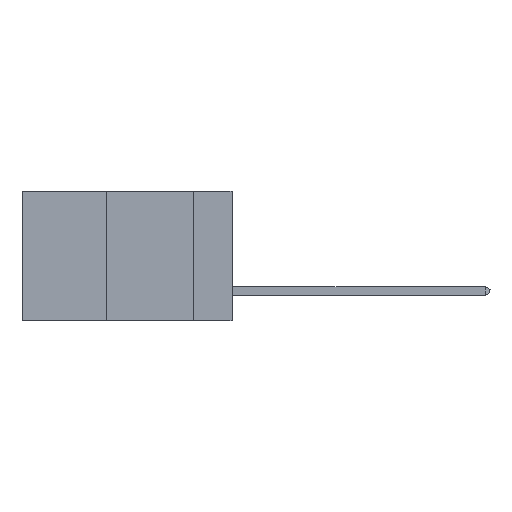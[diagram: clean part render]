
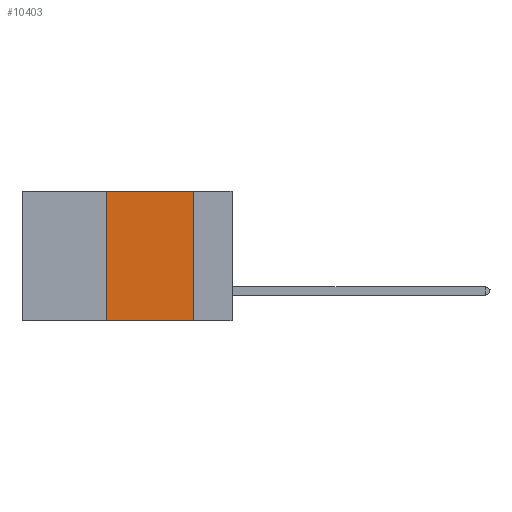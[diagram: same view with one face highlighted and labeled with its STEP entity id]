
A CAD part, left-side view. The second image highlights one B-rep face of the part: STEP entity #10403.
In plain terms, the highlighted planar face has unit normal (-1, 0, 0).
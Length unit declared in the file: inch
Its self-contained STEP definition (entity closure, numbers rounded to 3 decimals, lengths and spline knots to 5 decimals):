
#1484 = AXIS2_PLACEMENT_3D ( 'NONE', #18218, #8690, #34012 ) ;
#2479 = CARTESIAN_POINT ( 'NONE',  ( 0., 0.36, 0. ) ) ;
#2724 = CARTESIAN_POINT ( 'NONE',  ( 0., 0.6, -0.37 ) ) ;
#3680 = VERTEX_POINT ( 'NONE', #38893 ) ;
#3938 = DIRECTION ( 'NONE',  ( 0., -1., 0. ) ) ;
#5414 = VECTOR ( 'NONE', #3938, 39.37008 ) ;
#7353 = VECTOR ( 'NONE', #27477, 39.37008 ) ;
#7831 = LINE ( 'NONE', #2724, #7353 ) ;
#8361 = CARTESIAN_POINT ( 'NONE',  ( 0., 0.11, 0. ) ) ;
#8690 = DIRECTION ( 'NONE',  ( 1., 0., 0. ) ) ;
#10403 = ADVANCED_FACE ( 'NONE', ( #14463 ), #27562, .F. ) ;
#11799 = CARTESIAN_POINT ( 'NONE',  ( 0., 0.36, 0. ) ) ;
#12675 = VERTEX_POINT ( 'NONE', #37074 ) ;
#13739 = EDGE_LOOP ( 'NONE', ( #32101, #27097, #37524, #17548 ) ) ;
#14463 = FACE_OUTER_BOUND ( 'NONE', #13739, .T. ) ;
#17548 = ORIENTED_EDGE ( 'NONE', *, *, #30028, .T. ) ;
#18218 = CARTESIAN_POINT ( 'NONE',  ( 0., 0.6, 0. ) ) ;
#19046 = CARTESIAN_POINT ( 'NONE',  ( 0., 0.6, 0. ) ) ;
#19556 = EDGE_CURVE ( 'NONE', #34437, #36605, #22151, .T. ) ;
#19991 = CARTESIAN_POINT ( 'NONE',  ( 0., 0.11, 0. ) ) ;
#20805 = DIRECTION ( 'NONE',  ( 0., 0., -1. ) ) ;
#22151 = LINE ( 'NONE', #19046, #5414 ) ;
#25077 = EDGE_CURVE ( 'NONE', #12675, #34437, #33103, .T. ) ;
#27097 = ORIENTED_EDGE ( 'NONE', *, *, #19556, .F. ) ;
#27212 = VECTOR ( 'NONE', #27654, 39.37008 ) ;
#27477 = DIRECTION ( 'NONE',  ( 0., -1., 0. ) ) ;
#27562 = PLANE ( 'NONE',  #1484 ) ;
#27654 = DIRECTION ( 'NONE',  ( 0., 0., 1. ) ) ;
#28356 = LINE ( 'NONE', #8361, #37664 ) ;
#30028 = EDGE_CURVE ( 'NONE', #12675, #3680, #7831, .T. ) ;
#32101 = ORIENTED_EDGE ( 'NONE', *, *, #36170, .F. ) ;
#33103 = LINE ( 'NONE', #11799, #27212 ) ;
#34012 = DIRECTION ( 'NONE',  ( 0., 0., -1. ) ) ;
#34437 = VERTEX_POINT ( 'NONE', #2479 ) ;
#36170 = EDGE_CURVE ( 'NONE', #36605, #3680, #28356, .T. ) ;
#36605 = VERTEX_POINT ( 'NONE', #19991 ) ;
#37074 = CARTESIAN_POINT ( 'NONE',  ( 0., 0.36, -0.37 ) ) ;
#37524 = ORIENTED_EDGE ( 'NONE', *, *, #25077, .F. ) ;
#37664 = VECTOR ( 'NONE', #20805, 39.37008 ) ;
#38893 = CARTESIAN_POINT ( 'NONE',  ( 0., 0.11, -0.37 ) ) ;
